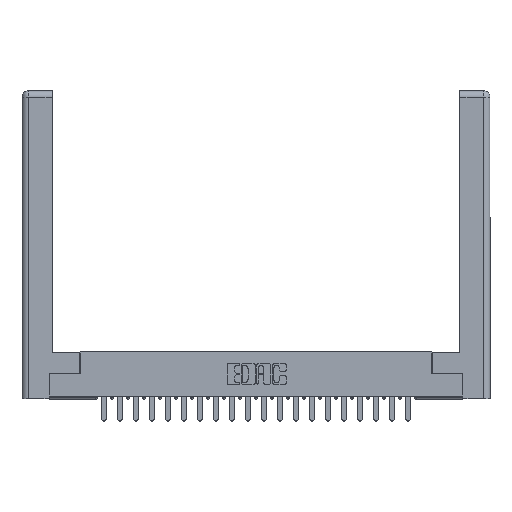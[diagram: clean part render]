
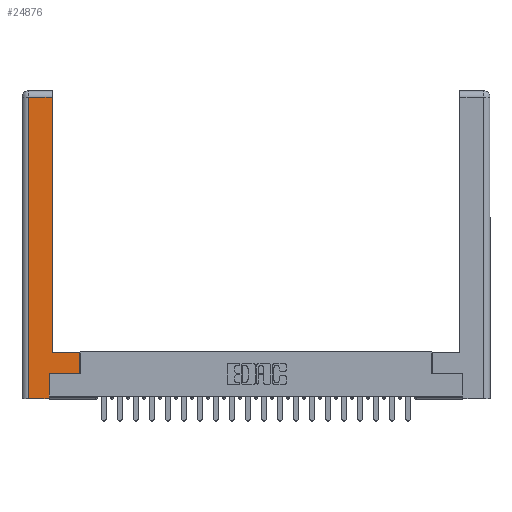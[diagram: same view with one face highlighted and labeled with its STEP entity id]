
A CAD part, top view. The second image highlights one B-rep face of the part: STEP entity #24876.
In plain terms, the highlighted planar face has unit normal (0, 0, 1).
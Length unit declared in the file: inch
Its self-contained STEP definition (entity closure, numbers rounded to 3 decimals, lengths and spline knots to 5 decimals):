
#12 = PLANE ( 'NONE',  #5774 ) ;
#94 = LINE ( 'NONE', #9675, #2705 ) ;
#908 = VERTEX_POINT ( 'NONE', #26050 ) ;
#1726 = CARTESIAN_POINT ( 'NONE',  ( 0., 0., 0. ) ) ;
#1881 = VERTEX_POINT ( 'NONE', #7276 ) ;
#2611 = VERTEX_POINT ( 'NONE', #3167 ) ;
#2631 = EDGE_CURVE ( 'NONE', #2611, #908, #6938, .T. ) ;
#2705 = VECTOR ( 'NONE', #18205, 39.37008 ) ;
#3167 = CARTESIAN_POINT ( 'NONE',  ( 0.295, 2.94, 0. ) ) ;
#3313 = VECTOR ( 'NONE', #5584, 39.37008 ) ;
#3454 = LINE ( 'NONE', #19261, #20913 ) ;
#3517 = CARTESIAN_POINT ( 'NONE',  ( 0.0615, 2.94, 0. ) ) ;
#3602 = CARTESIAN_POINT ( 'NONE',  ( 0.0615, 0., 0. ) ) ;
#4387 = ORIENTED_EDGE ( 'NONE', *, *, #9488, .T. ) ;
#4813 = DIRECTION ( 'NONE',  ( 0., 1., 0. ) ) ;
#5331 = VECTOR ( 'NONE', #4813, 39.37008 ) ;
#5554 = CARTESIAN_POINT ( 'NONE',  ( 0.565, 0.245, 0. ) ) ;
#5584 = DIRECTION ( 'NONE',  ( 0., -1., 0. ) ) ;
#5618 = ORIENTED_EDGE ( 'NONE', *, *, #13347, .T. ) ;
#5774 = AXIS2_PLACEMENT_3D ( 'NONE', #1726, #18472, #10358 ) ;
#6677 = EDGE_CURVE ( 'NONE', #7468, #25582, #18469, .T. ) ;
#6938 = LINE ( 'NONE', #3517, #15951 ) ;
#7276 = CARTESIAN_POINT ( 'NONE',  ( 0.295, 0.45, 0. ) ) ;
#7468 = VERTEX_POINT ( 'NONE', #22041 ) ;
#7497 = VECTOR ( 'NONE', #16503, 39.37008 ) ;
#8407 = CARTESIAN_POINT ( 'NONE',  ( 0.265, 0.245, 0. ) ) ;
#8775 = ORIENTED_EDGE ( 'NONE', *, *, #21637, .T. ) ;
#8800 = ORIENTED_EDGE ( 'NONE', *, *, #2631, .T. ) ;
#9168 = DIRECTION ( 'NONE',  ( 0., 1., 0. ) ) ;
#9488 = EDGE_CURVE ( 'NONE', #23559, #7468, #94, .T. ) ;
#9675 = CARTESIAN_POINT ( 'NONE',  ( 0.265, 0., 0. ) ) ;
#10292 = ORIENTED_EDGE ( 'NONE', *, *, #25589, .T. ) ;
#10358 = DIRECTION ( 'NONE',  ( -1., 0., 0. ) ) ;
#10567 = CARTESIAN_POINT ( 'NONE',  ( 0.0615, 0., 0. ) ) ;
#10683 = ORIENTED_EDGE ( 'NONE', *, *, #6677, .T. ) ;
#10733 = CARTESIAN_POINT ( 'NONE',  ( 0.295, 3., 0. ) ) ;
#10870 = LINE ( 'NONE', #10733, #5331 ) ;
#13347 = EDGE_CURVE ( 'NONE', #20653, #1881, #3454, .T. ) ;
#14213 = VECTOR ( 'NONE', #9168, 39.37008 ) ;
#14626 = ORIENTED_EDGE ( 'NONE', *, *, #17180, .T. ) ;
#15073 = DIRECTION ( 'NONE',  ( -1., 0., 0. ) ) ;
#15150 = FACE_OUTER_BOUND ( 'NONE', #24448, .T. ) ;
#15951 = VECTOR ( 'NONE', #26183, 39.37008 ) ;
#16503 = DIRECTION ( 'NONE',  ( 0., 1., 0. ) ) ;
#17180 = EDGE_CURVE ( 'NONE', #25582, #21283, #23615, .T. ) ;
#17206 = LINE ( 'NONE', #3602, #3313 ) ;
#18205 = DIRECTION ( 'NONE',  ( 1., 0., 0. ) ) ;
#18469 = LINE ( 'NONE', #8407, #7497 ) ;
#18472 = DIRECTION ( 'NONE',  ( 0., 0., -1. ) ) ;
#19261 = CARTESIAN_POINT ( 'NONE',  ( 0.295, 0.45, 0. ) ) ;
#19349 = VECTOR ( 'NONE', #22511, 39.37008 ) ;
#19703 = LINE ( 'NONE', #23731, #14213 ) ;
#20119 = CARTESIAN_POINT ( 'NONE',  ( 0.565, 0.45, 0. ) ) ;
#20583 = CARTESIAN_POINT ( 'NONE',  ( 0.565, 0.245, 0. ) ) ;
#20653 = VERTEX_POINT ( 'NONE', #20119 ) ;
#20913 = VECTOR ( 'NONE', #15073, 39.37008 ) ;
#21283 = VERTEX_POINT ( 'NONE', #5554 ) ;
#21637 = EDGE_CURVE ( 'NONE', #1881, #2611, #10870, .T. ) ;
#22041 = CARTESIAN_POINT ( 'NONE',  ( 0.265, 0., 0. ) ) ;
#22511 = DIRECTION ( 'NONE',  ( 1., 0., 0. ) ) ;
#23306 = EDGE_CURVE ( 'NONE', #908, #23559, #17206, .T. ) ;
#23556 = CARTESIAN_POINT ( 'NONE',  ( 0.265, 0.245, 0. ) ) ;
#23559 = VERTEX_POINT ( 'NONE', #10567 ) ;
#23615 = LINE ( 'NONE', #20583, #19349 ) ;
#23731 = CARTESIAN_POINT ( 'NONE',  ( 0.565, 0.45, 0. ) ) ;
#24347 = ORIENTED_EDGE ( 'NONE', *, *, #23306, .T. ) ;
#24448 = EDGE_LOOP ( 'NONE', ( #8775, #8800, #24347, #4387, #10683, #14626, #10292, #5618 ) ) ;
#24876 = ADVANCED_FACE ( 'NONE', ( #15150 ), #12, .F. ) ;
#25582 = VERTEX_POINT ( 'NONE', #23556 ) ;
#25589 = EDGE_CURVE ( 'NONE', #21283, #20653, #19703, .T. ) ;
#26050 = CARTESIAN_POINT ( 'NONE',  ( 0.0615, 2.94, 0. ) ) ;
#26183 = DIRECTION ( 'NONE',  ( -1., 0., 0. ) ) ;
